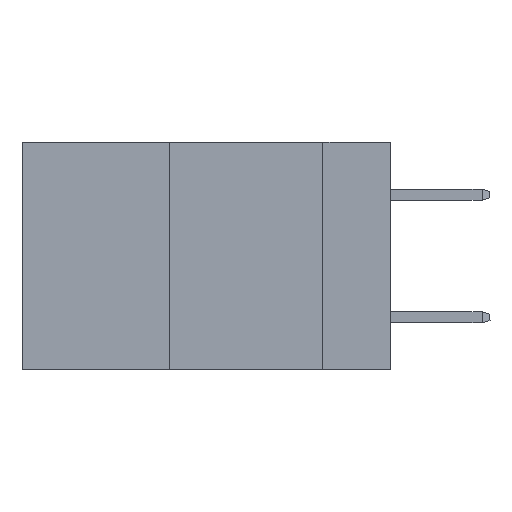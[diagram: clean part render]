
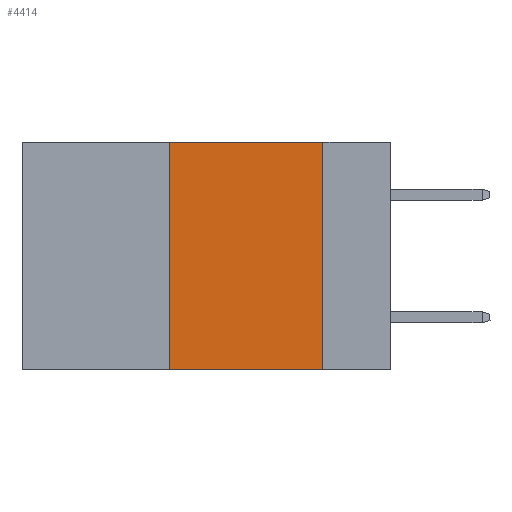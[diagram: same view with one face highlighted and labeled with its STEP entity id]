
A CAD part, left-side view. The second image highlights one B-rep face of the part: STEP entity #4414.
In plain terms, the highlighted planar face has unit normal (-1, 0, 0).
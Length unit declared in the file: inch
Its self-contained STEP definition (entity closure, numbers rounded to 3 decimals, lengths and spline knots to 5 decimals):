
#1129 = EDGE_LOOP ( 'NONE', ( #16477, #1957, #8249, #13859 ) ) ;
#1432 = CARTESIAN_POINT ( 'NONE',  ( 0., 0.6, 0. ) ) ;
#1957 = ORIENTED_EDGE ( 'NONE', *, *, #13849, .F. ) ;
#2296 = CARTESIAN_POINT ( 'NONE',  ( 0., 0.6, 0. ) ) ;
#2541 = LINE ( 'NONE', #17098, #13680 ) ;
#2824 = LINE ( 'NONE', #9762, #6248 ) ;
#3784 = DIRECTION ( 'NONE',  ( 0., 0., -1. ) ) ;
#4027 = AXIS2_PLACEMENT_3D ( 'NONE', #2296, #12498, #3784 ) ;
#4414 = ADVANCED_FACE ( 'NONE', ( #8647 ), #5191, .F. ) ;
#4886 = CARTESIAN_POINT ( 'NONE',  ( 0., 0.11, 0. ) ) ;
#5191 = PLANE ( 'NONE',  #4027 ) ;
#5461 = VERTEX_POINT ( 'NONE', #4886 ) ;
#5985 = DIRECTION ( 'NONE',  ( 0., -1., 0. ) ) ;
#6248 = VECTOR ( 'NONE', #15455, 39.37008 ) ;
#6755 = VECTOR ( 'NONE', #5985, 39.37008 ) ;
#7212 = CARTESIAN_POINT ( 'NONE',  ( 0., 0.36, -0.37 ) ) ;
#7498 = EDGE_CURVE ( 'NONE', #18716, #15612, #2541, .T. ) ;
#8249 = ORIENTED_EDGE ( 'NONE', *, *, #7498, .F. ) ;
#8647 = FACE_OUTER_BOUND ( 'NONE', #1129, .T. ) ;
#9610 = DIRECTION ( 'NONE',  ( 0., 0., -1. ) ) ;
#9762 = CARTESIAN_POINT ( 'NONE',  ( 0., 0.6, -0.37 ) ) ;
#10070 = DIRECTION ( 'NONE',  ( 0., 0., 1. ) ) ;
#10428 = EDGE_CURVE ( 'NONE', #5461, #18523, #15783, .T. ) ;
#11099 = CARTESIAN_POINT ( 'NONE',  ( 0., 0.11, 0. ) ) ;
#12060 = VECTOR ( 'NONE', #9610, 39.37008 ) ;
#12498 = DIRECTION ( 'NONE',  ( 1., 0., 0. ) ) ;
#13680 = VECTOR ( 'NONE', #10070, 39.37008 ) ;
#13849 = EDGE_CURVE ( 'NONE', #15612, #5461, #14384, .T. ) ;
#13859 = ORIENTED_EDGE ( 'NONE', *, *, #14259, .T. ) ;
#14259 = EDGE_CURVE ( 'NONE', #18716, #18523, #2824, .T. ) ;
#14380 = CARTESIAN_POINT ( 'NONE',  ( 0., 0.36, 0. ) ) ;
#14384 = LINE ( 'NONE', #1432, #6755 ) ;
#15455 = DIRECTION ( 'NONE',  ( 0., -1., 0. ) ) ;
#15612 = VERTEX_POINT ( 'NONE', #14380 ) ;
#15783 = LINE ( 'NONE', #11099, #12060 ) ;
#16477 = ORIENTED_EDGE ( 'NONE', *, *, #10428, .F. ) ;
#16566 = CARTESIAN_POINT ( 'NONE',  ( 0., 0.11, -0.37 ) ) ;
#17098 = CARTESIAN_POINT ( 'NONE',  ( 0., 0.36, 0. ) ) ;
#18523 = VERTEX_POINT ( 'NONE', #16566 ) ;
#18716 = VERTEX_POINT ( 'NONE', #7212 ) ;
